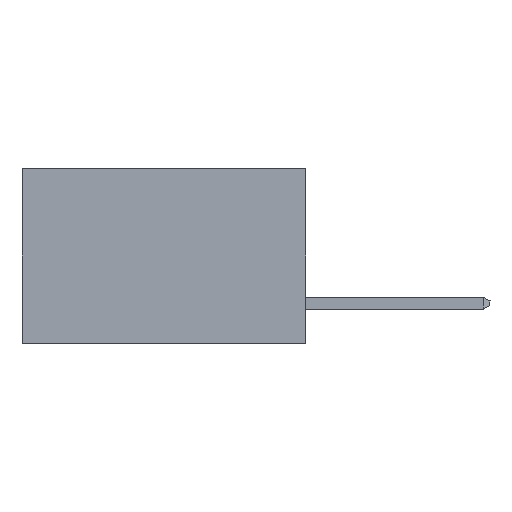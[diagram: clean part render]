
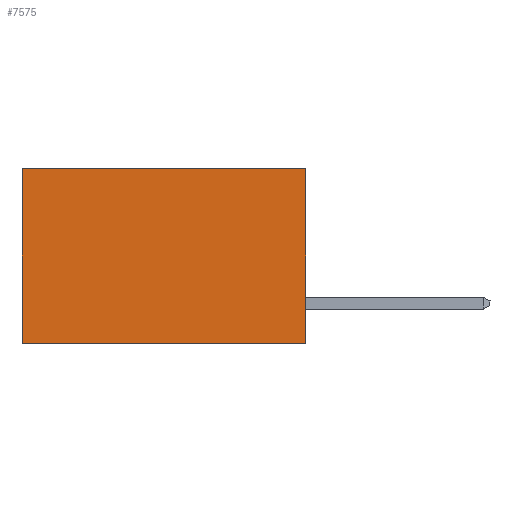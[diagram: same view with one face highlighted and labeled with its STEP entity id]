
A CAD part, left-side view. The second image highlights one B-rep face of the part: STEP entity #7575.
In plain terms, the highlighted planar face has unit normal (-1, 0, 0).
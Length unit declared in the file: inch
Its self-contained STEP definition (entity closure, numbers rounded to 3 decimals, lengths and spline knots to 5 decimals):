
#385 = CARTESIAN_POINT ( 'NONE',  ( 0.298, 0.6, 0. ) ) ;
#3222 = CARTESIAN_POINT ( 'NONE',  ( 0.298, 0., 0. ) ) ;
#3483 = VECTOR ( 'NONE', #7501, 39.37008 ) ;
#5423 = EDGE_CURVE ( 'NONE', #21160, #21820, #11231, .T. ) ;
#6322 = VECTOR ( 'NONE', #24533, 39.37008 ) ;
#6823 = DIRECTION ( 'NONE',  ( 0., 0., -1. ) ) ;
#7360 = CARTESIAN_POINT ( 'NONE',  ( 0.298, 0.6, 0. ) ) ;
#7501 = DIRECTION ( 'NONE',  ( 0., 0., -1. ) ) ;
#7575 = ADVANCED_FACE ( 'NONE', ( #25806 ), #20387, .F. ) ;
#8720 = LINE ( 'NONE', #13493, #22712 ) ;
#8958 = ORIENTED_EDGE ( 'NONE', *, *, #5423, .T. ) ;
#9507 = EDGE_CURVE ( 'NONE', #10509, #21820, #22509, .T. ) ;
#10509 = VERTEX_POINT ( 'NONE', #12231 ) ;
#11231 = LINE ( 'NONE', #7360, #11945 ) ;
#11945 = VECTOR ( 'NONE', #28044, 39.37008 ) ;
#12202 = AXIS2_PLACEMENT_3D ( 'NONE', #13689, #29685, #6823 ) ;
#12231 = CARTESIAN_POINT ( 'NONE',  ( 0.298, 0., -0.37 ) ) ;
#13493 = CARTESIAN_POINT ( 'NONE',  ( 0.298, 0., 0. ) ) ;
#13538 = EDGE_LOOP ( 'NONE', ( #8958, #25708, #23390, #24541 ) ) ;
#13689 = CARTESIAN_POINT ( 'NONE',  ( 0.298, 0., 0. ) ) ;
#15899 = DIRECTION ( 'NONE',  ( 0., 1., 0. ) ) ;
#16453 = CARTESIAN_POINT ( 'NONE',  ( 0.298, 0.6, -0.37 ) ) ;
#17961 = LINE ( 'NONE', #25587, #3483 ) ;
#20387 = PLANE ( 'NONE',  #12202 ) ;
#21160 = VERTEX_POINT ( 'NONE', #385 ) ;
#21820 = VERTEX_POINT ( 'NONE', #16453 ) ;
#21913 = VERTEX_POINT ( 'NONE', #3222 ) ;
#22509 = LINE ( 'NONE', #28945, #6322 ) ;
#22712 = VECTOR ( 'NONE', #15899, 39.37008 ) ;
#23390 = ORIENTED_EDGE ( 'NONE', *, *, #28789, .F. ) ;
#24533 = DIRECTION ( 'NONE',  ( 0., 1., 0. ) ) ;
#24541 = ORIENTED_EDGE ( 'NONE', *, *, #26508, .T. ) ;
#25587 = CARTESIAN_POINT ( 'NONE',  ( 0.298, 0., 0. ) ) ;
#25708 = ORIENTED_EDGE ( 'NONE', *, *, #9507, .F. ) ;
#25806 = FACE_OUTER_BOUND ( 'NONE', #13538, .T. ) ;
#26508 = EDGE_CURVE ( 'NONE', #21913, #21160, #8720, .T. ) ;
#28044 = DIRECTION ( 'NONE',  ( 0., 0., -1. ) ) ;
#28789 = EDGE_CURVE ( 'NONE', #21913, #10509, #17961, .T. ) ;
#28945 = CARTESIAN_POINT ( 'NONE',  ( 0.298, 0., -0.37 ) ) ;
#29685 = DIRECTION ( 'NONE',  ( 1., 0., 0. ) ) ;
